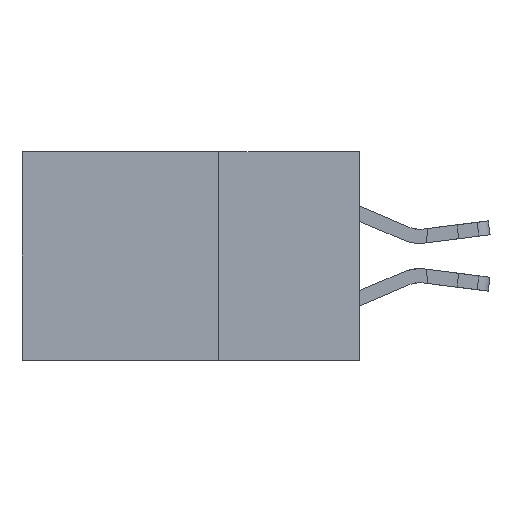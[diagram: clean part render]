
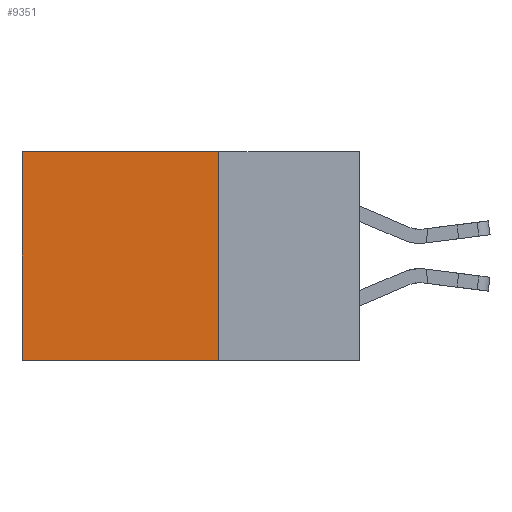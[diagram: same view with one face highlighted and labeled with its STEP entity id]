
A CAD part, left-side view. The second image highlights one B-rep face of the part: STEP entity #9351.
In plain terms, the highlighted planar face has unit normal (-1, 0, 0).
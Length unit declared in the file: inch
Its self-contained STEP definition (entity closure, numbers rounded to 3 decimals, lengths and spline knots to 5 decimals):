
#455 = DIRECTION ( 'NONE',  ( 0., 0., -1. ) ) ;
#1122 = EDGE_CURVE ( 'NONE', #10102, #11560, #32152, .T. ) ;
#1149 = CARTESIAN_POINT ( 'NONE',  ( 0.2875, 0.6, -0.37 ) ) ;
#1412 = LINE ( 'NONE', #32224, #26143 ) ;
#3689 = CARTESIAN_POINT ( 'NONE',  ( 0.2875, 0.6, 0. ) ) ;
#3886 = VERTEX_POINT ( 'NONE', #23910 ) ;
#4090 = DIRECTION ( 'NONE',  ( 0., 1., 0. ) ) ;
#5014 = CARTESIAN_POINT ( 'NONE',  ( 0.2875, 0.6, 0. ) ) ;
#5033 = VECTOR ( 'NONE', #455, 39.37008 ) ;
#5981 = PLANE ( 'NONE',  #6629 ) ;
#6629 = AXIS2_PLACEMENT_3D ( 'NONE', #8507, #16024, #8675 ) ;
#7752 = ORIENTED_EDGE ( 'NONE', *, *, #9277, .F. ) ;
#8507 = CARTESIAN_POINT ( 'NONE',  ( 0.2875, 0.25, 0. ) ) ;
#8675 = DIRECTION ( 'NONE',  ( 0., 0., -1. ) ) ;
#9060 = ORIENTED_EDGE ( 'NONE', *, *, #29035, .F. ) ;
#9277 = EDGE_CURVE ( 'NONE', #23222, #3886, #10347, .T. ) ;
#9351 = ADVANCED_FACE ( 'NONE', ( #26224 ), #5981, .F. ) ;
#9738 = ORIENTED_EDGE ( 'NONE', *, *, #1122, .T. ) ;
#10102 = VERTEX_POINT ( 'NONE', #5014 ) ;
#10347 = LINE ( 'NONE', #13200, #5033 ) ;
#11560 = VERTEX_POINT ( 'NONE', #1149 ) ;
#12103 = VECTOR ( 'NONE', #19587, 39.37008 ) ;
#13200 = CARTESIAN_POINT ( 'NONE',  ( 0.2875, 0.25, 0. ) ) ;
#16024 = DIRECTION ( 'NONE',  ( 1., 0., 0. ) ) ;
#16275 = CARTESIAN_POINT ( 'NONE',  ( 0.2875, 0.25, 0. ) ) ;
#16335 = EDGE_LOOP ( 'NONE', ( #9738, #9060, #7752, #21807 ) ) ;
#19587 = DIRECTION ( 'NONE',  ( 0., 0., -1. ) ) ;
#21807 = ORIENTED_EDGE ( 'NONE', *, *, #23590, .T. ) ;
#21937 = LINE ( 'NONE', #16275, #27576 ) ;
#23222 = VERTEX_POINT ( 'NONE', #30191 ) ;
#23590 = EDGE_CURVE ( 'NONE', #23222, #10102, #21937, .T. ) ;
#23910 = CARTESIAN_POINT ( 'NONE',  ( 0.2875, 0.25, -0.37 ) ) ;
#26143 = VECTOR ( 'NONE', #4090, 39.37008 ) ;
#26224 = FACE_OUTER_BOUND ( 'NONE', #16335, .T. ) ;
#26477 = DIRECTION ( 'NONE',  ( 0., 1., 0. ) ) ;
#27576 = VECTOR ( 'NONE', #26477, 39.37008 ) ;
#29035 = EDGE_CURVE ( 'NONE', #3886, #11560, #1412, .T. ) ;
#30191 = CARTESIAN_POINT ( 'NONE',  ( 0.2875, 0.25, 0. ) ) ;
#32152 = LINE ( 'NONE', #3689, #12103 ) ;
#32224 = CARTESIAN_POINT ( 'NONE',  ( 0.2875, 0.25, -0.37 ) ) ;
